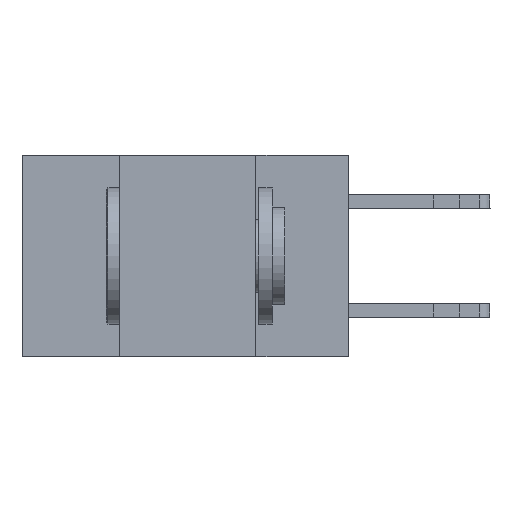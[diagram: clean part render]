
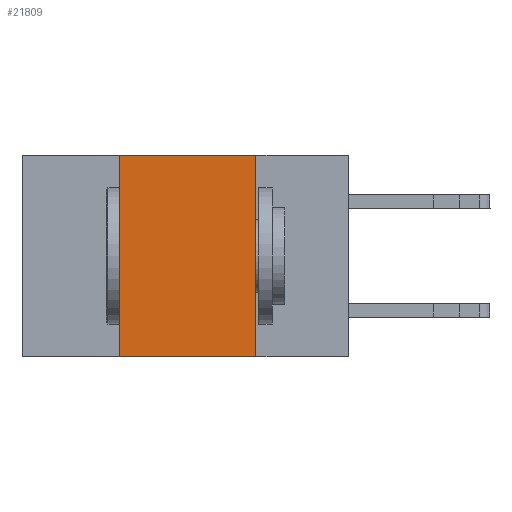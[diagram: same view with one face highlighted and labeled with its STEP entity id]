
A CAD part, left-side view. The second image highlights one B-rep face of the part: STEP entity #21809.
In plain terms, the highlighted planar face has unit normal (-1, 0, 0).
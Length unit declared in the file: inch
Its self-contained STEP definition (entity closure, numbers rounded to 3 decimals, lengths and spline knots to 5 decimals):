
#337 = EDGE_CURVE ( 'NONE', #20401, #13535, #2463, .T. ) ;
#491 = ORIENTED_EDGE ( 'NONE', *, *, #6839, .F. ) ;
#1709 = DIRECTION ( 'NONE',  ( 0., -1., 0. ) ) ;
#1745 = VERTEX_POINT ( 'NONE', #11703 ) ;
#2463 = LINE ( 'NONE', #6535, #23594 ) ;
#4182 = CARTESIAN_POINT ( 'NONE',  ( 0., 0.42, -0.37 ) ) ;
#4473 = LINE ( 'NONE', #22692, #12601 ) ;
#4815 = VECTOR ( 'NONE', #12351, 39.37008 ) ;
#5560 = ORIENTED_EDGE ( 'NONE', *, *, #6177, .F. ) ;
#6177 = EDGE_CURVE ( 'NONE', #14158, #1745, #19750, .T. ) ;
#6535 = CARTESIAN_POINT ( 'NONE',  ( 0., 0.42, -0.37 ) ) ;
#6839 = EDGE_CURVE ( 'NONE', #13535, #14158, #9144, .T. ) ;
#7272 = CARTESIAN_POINT ( 'NONE',  ( 0., 0.17, 0. ) ) ;
#7452 = ORIENTED_EDGE ( 'NONE', *, *, #13125, .T. ) ;
#7794 = FACE_OUTER_BOUND ( 'NONE', #23169, .T. ) ;
#8255 = CARTESIAN_POINT ( 'NONE',  ( 0., 0.6, 0. ) ) ;
#9144 = LINE ( 'NONE', #15014, #14895 ) ;
#10135 = DIRECTION ( 'NONE',  ( 0., 0., 1. ) ) ;
#10664 = CARTESIAN_POINT ( 'NONE',  ( 0., 0.17, -0.37 ) ) ;
#11446 = AXIS2_PLACEMENT_3D ( 'NONE', #8255, #15104, #18917 ) ;
#11685 = DIRECTION ( 'NONE',  ( 0., -1., 0. ) ) ;
#11703 = CARTESIAN_POINT ( 'NONE',  ( 0., 0.17, -0.37 ) ) ;
#11894 = CARTESIAN_POINT ( 'NONE',  ( 0., 0.42, 0. ) ) ;
#12351 = DIRECTION ( 'NONE',  ( 0., 0., -1. ) ) ;
#12601 = VECTOR ( 'NONE', #11685, 39.37008 ) ;
#13125 = EDGE_CURVE ( 'NONE', #20401, #1745, #4473, .T. ) ;
#13535 = VERTEX_POINT ( 'NONE', #11894 ) ;
#14158 = VERTEX_POINT ( 'NONE', #7272 ) ;
#14895 = VECTOR ( 'NONE', #1709, 39.37008 ) ;
#15014 = CARTESIAN_POINT ( 'NONE',  ( 0., 0.6, 0. ) ) ;
#15104 = DIRECTION ( 'NONE',  ( 1., 0., 0. ) ) ;
#17368 = ORIENTED_EDGE ( 'NONE', *, *, #337, .F. ) ;
#18917 = DIRECTION ( 'NONE',  ( 0., 0., -1. ) ) ;
#19750 = LINE ( 'NONE', #10664, #4815 ) ;
#20401 = VERTEX_POINT ( 'NONE', #4182 ) ;
#21809 = ADVANCED_FACE ( 'NONE', ( #7794 ), #22514, .F. ) ;
#22514 = PLANE ( 'NONE',  #11446 ) ;
#22692 = CARTESIAN_POINT ( 'NONE',  ( 0., 0.6, -0.37 ) ) ;
#23169 = EDGE_LOOP ( 'NONE', ( #5560, #491, #17368, #7452 ) ) ;
#23594 = VECTOR ( 'NONE', #10135, 39.37008 ) ;
